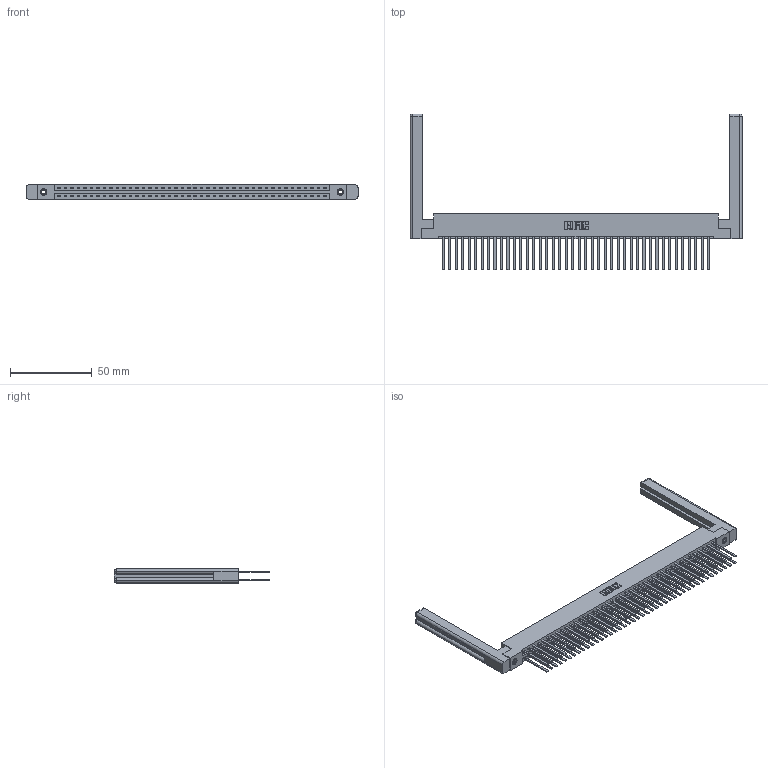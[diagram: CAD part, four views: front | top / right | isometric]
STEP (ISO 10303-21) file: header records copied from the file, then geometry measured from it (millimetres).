
FILE_DESCRIPTION (( 'STEP AP203' ), '1' );
FILE_NAME ('337-084-544-258.STEP', '2019-10-10T14:11:52', ( '' ), ( '' ), 'SwSTEP 2.0', 'SolidWorks 2016', '' );
FILE_SCHEMA (( 'CONFIG_CONTROL_DESIGN' ));
Length unit declared in the file: inch
Products named in the file (5): 307-220-058; 345-292-001_345-293-144; 337-084-544-258; 337 Part_Flush Mounting Lugs - 0.156 Dia-TI; 345-250-001_345-250-001-102
Assembly tree (89 placements, depth 2):
  337-084-544-258
    337 Part_Flush Mounting Lugs - 0.156 Dia-TI
    345-292-001_345-293-144  x84
    345-250-001_345-250-001-102  x2
    307-220-058  x2
Bounding box: 203.05 x 95.38 x 9.4 mm (x, y, z)
Volume: 29718.6 mm3; surface area: 34416 mm2
Topology: 89 solids, 89 shells, 4288 faces, 12677 edges, 8326 vertices
Faces by surface type: plane 3010, cylinder 1254, cone 12, torus 12
Entity records: 35014 total; most frequent: CARTESIAN_POINT 5905, ORIENTED_EDGE 5780, DIRECTION 5034, EDGE_CURVE 2890, VECTOR 2718, LINE 2718, VERTEX_POINT 1918, AXIS2_PLACEMENT_3D 1158
